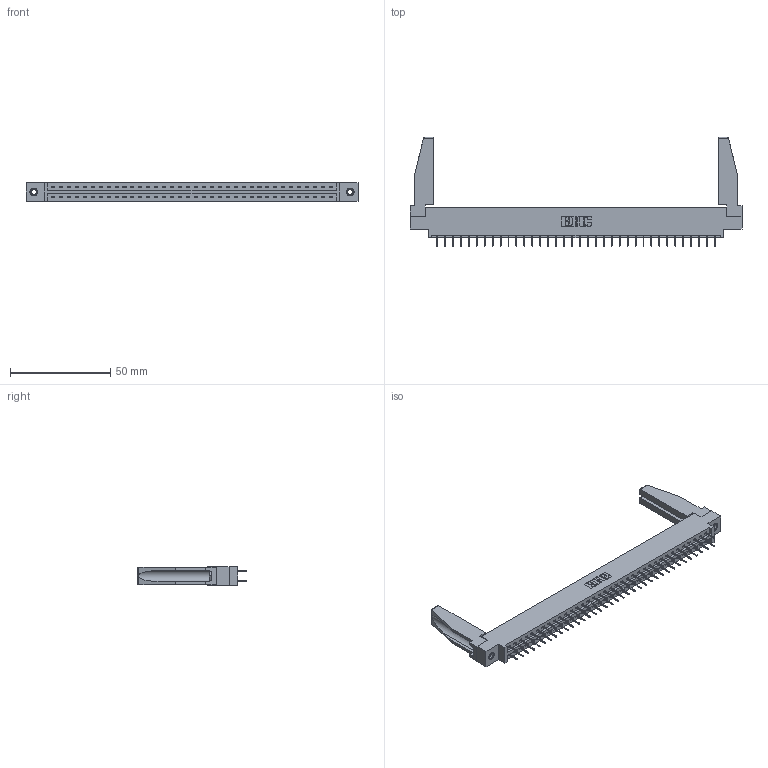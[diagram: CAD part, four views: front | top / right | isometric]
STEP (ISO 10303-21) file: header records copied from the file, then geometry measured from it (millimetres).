
FILE_DESCRIPTION (( 'STEP AP203' ), '1' );
FILE_NAME ('387-072-524-878.STEP', '2019-10-21T23:50:28', ( '' ), ( '' ), 'SwSTEP 2.0', 'SolidWorks 2016', '' );
FILE_SCHEMA (( 'CONFIG_CONTROL_DESIGN' ));
Length unit declared in the file: inch
Products named in the file (5): 337 Part_0.170 Offset - 0.156 Dia-TI; 387-072-524-878; 345-292-001_345-293-124; 307-220-078; 345-250-001_345-250-001-102
Assembly tree (77 placements, depth 2):
  387-072-524-878
    337 Part_0.170 Offset - 0.156 Dia-TI
    345-292-001_345-293-124  x72
    345-250-001_345-250-001-102  x2
    307-220-078  x2
Bounding box: 165.66 x 54.49 x 9.4 mm (x, y, z)
Volume: 21145.4 mm3; surface area: 22933 mm2
Topology: 77 solids, 77 shells, 4424 faces, 12533 edges, 8058 vertices
Faces by surface type: plane 3326, cylinder 1082, cone 12, torus 4
Entity records: 31334 total; most frequent: CARTESIAN_POINT 5284, ORIENTED_EDGE 5176, DIRECTION 4512, EDGE_CURVE 2588, VECTOR 2426, LINE 2426, VERTEX_POINT 1716, AXIS2_PLACEMENT_3D 1043
